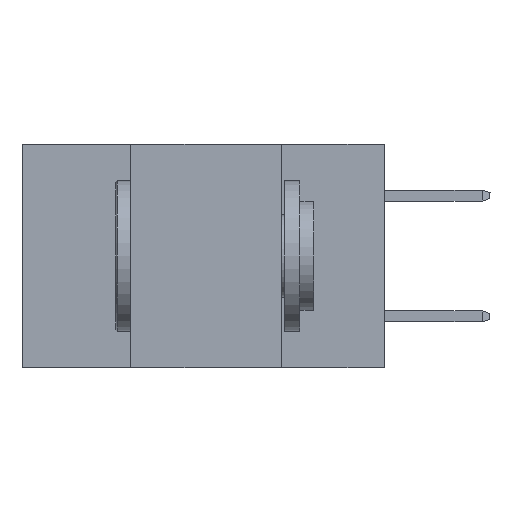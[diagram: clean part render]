
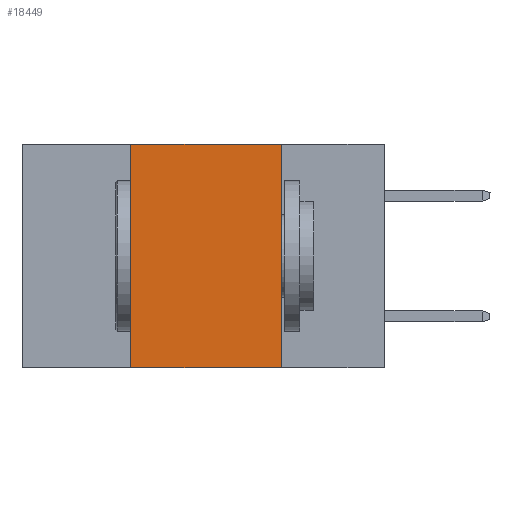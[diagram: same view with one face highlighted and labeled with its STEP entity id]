
A CAD part, left-side view. The second image highlights one B-rep face of the part: STEP entity #18449.
In plain terms, the highlighted planar face has unit normal (-1, 0, 0).
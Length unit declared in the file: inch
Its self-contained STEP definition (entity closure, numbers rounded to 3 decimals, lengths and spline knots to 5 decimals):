
#8 = EDGE_CURVE ( 'NONE', #20113, #13940, #24171, .T. ) ;
#312 = VERTEX_POINT ( 'NONE', #15456 ) ;
#826 = CARTESIAN_POINT ( 'NONE',  ( 0., 0.6, -0.37 ) ) ;
#1174 = DIRECTION ( 'NONE',  ( 0., -1., 0. ) ) ;
#1210 = FACE_OUTER_BOUND ( 'NONE', #3203, .T. ) ;
#2112 = VECTOR ( 'NONE', #1174, 39.37008 ) ;
#2629 = VECTOR ( 'NONE', #4814, 39.37008 ) ;
#3003 = LINE ( 'NONE', #826, #18009 ) ;
#3042 = CARTESIAN_POINT ( 'NONE',  ( 0., 0.42, -0.37 ) ) ;
#3203 = EDGE_LOOP ( 'NONE', ( #22188, #14903, #12437, #22978 ) ) ;
#4814 = DIRECTION ( 'NONE',  ( 0., 0., 1. ) ) ;
#6769 = CARTESIAN_POINT ( 'NONE',  ( 0., 0.6, 0. ) ) ;
#6952 = PLANE ( 'NONE',  #20080 ) ;
#8834 = DIRECTION ( 'NONE',  ( 1., 0., 0. ) ) ;
#10972 = LINE ( 'NONE', #6769, #2112 ) ;
#12437 = ORIENTED_EDGE ( 'NONE', *, *, #21895, .F. ) ;
#12655 = CARTESIAN_POINT ( 'NONE',  ( 0., 0.6, 0. ) ) ;
#13791 = DIRECTION ( 'NONE',  ( 0., -1., 0. ) ) ;
#13914 = EDGE_CURVE ( 'NONE', #312, #20113, #10972, .T. ) ;
#13940 = VERTEX_POINT ( 'NONE', #24105 ) ;
#14197 = VECTOR ( 'NONE', #15509, 39.37008 ) ;
#14538 = DIRECTION ( 'NONE',  ( 0., 0., -1. ) ) ;
#14903 = ORIENTED_EDGE ( 'NONE', *, *, #13914, .F. ) ;
#15456 = CARTESIAN_POINT ( 'NONE',  ( 0., 0.42, 0. ) ) ;
#15509 = DIRECTION ( 'NONE',  ( 0., 0., -1. ) ) ;
#15900 = LINE ( 'NONE', #21646, #2629 ) ;
#17133 = EDGE_CURVE ( 'NONE', #18829, #13940, #3003, .T. ) ;
#18009 = VECTOR ( 'NONE', #13791, 39.37008 ) ;
#18449 = ADVANCED_FACE ( 'NONE', ( #1210 ), #6952, .F. ) ;
#18829 = VERTEX_POINT ( 'NONE', #3042 ) ;
#20080 = AXIS2_PLACEMENT_3D ( 'NONE', #12655, #8834, #14538 ) ;
#20113 = VERTEX_POINT ( 'NONE', #21959 ) ;
#21646 = CARTESIAN_POINT ( 'NONE',  ( 0., 0.42, 0. ) ) ;
#21895 = EDGE_CURVE ( 'NONE', #18829, #312, #15900, .T. ) ;
#21959 = CARTESIAN_POINT ( 'NONE',  ( 0., 0.17, 0. ) ) ;
#22188 = ORIENTED_EDGE ( 'NONE', *, *, #8, .F. ) ;
#22966 = CARTESIAN_POINT ( 'NONE',  ( 0., 0.17, 0. ) ) ;
#22978 = ORIENTED_EDGE ( 'NONE', *, *, #17133, .T. ) ;
#24105 = CARTESIAN_POINT ( 'NONE',  ( 0., 0.17, -0.37 ) ) ;
#24171 = LINE ( 'NONE', #22966, #14197 ) ;
